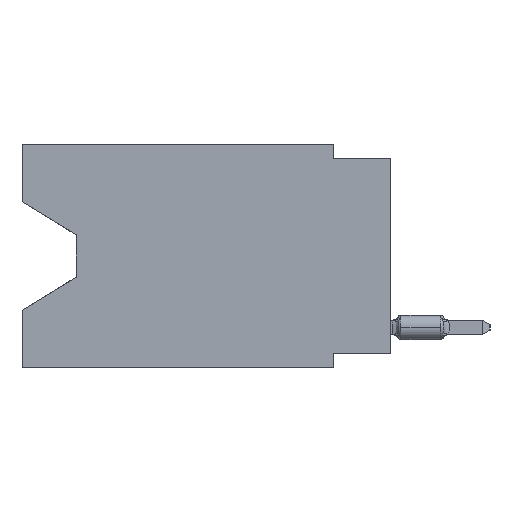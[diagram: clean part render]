
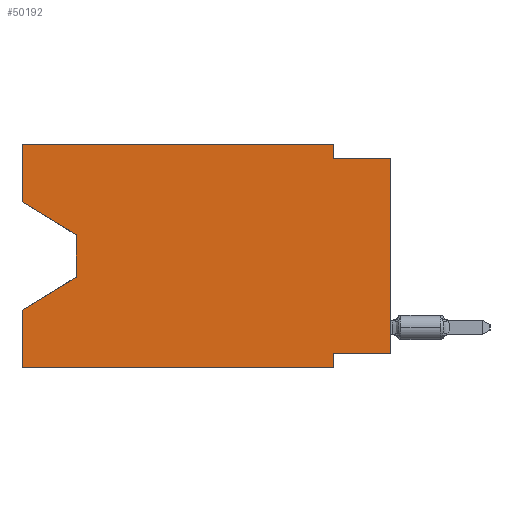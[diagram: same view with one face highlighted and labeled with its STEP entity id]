
A CAD part, left-side view. The second image highlights one B-rep face of the part: STEP entity #50192.
In plain terms, the highlighted planar face has unit normal (-1, 0, 0).
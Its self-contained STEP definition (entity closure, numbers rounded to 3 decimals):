
#1399 = ORIENTED_EDGE ( 'NONE', *, *, #29018, .T. ) ;
#1753 = CARTESIAN_POINT ( 'NONE',  ( 0., 13.97, -5.893 ) ) ;
#2092 = CARTESIAN_POINT ( 'NONE',  ( 0., 16.383, 0. ) ) ;
#2249 = EDGE_CURVE ( 'NONE', #56147, #43736, #60631, .T. ) ;
#2749 = LINE ( 'NONE', #41921, #39977 ) ;
#3584 = AXIS2_PLACEMENT_3D ( 'NONE', #2092, #50902, #56037 ) ;
#4312 = CARTESIAN_POINT ( 'NONE',  ( 0., 2.54, -9.906 ) ) ;
#4635 = VERTEX_POINT ( 'NONE', #38450 ) ;
#6083 = LINE ( 'NONE', #30810, #52205 ) ;
#6683 = DIRECTION ( 'NONE',  ( 0., 0., -1. ) ) ;
#8539 = EDGE_CURVE ( 'NONE', #33124, #56147, #19864, .T. ) ;
#9838 = LINE ( 'NONE', #18857, #56241 ) ;
#11306 = CARTESIAN_POINT ( 'NONE',  ( 0., 2.54, -0.635 ) ) ;
#11333 = CARTESIAN_POINT ( 'NONE',  ( 0., 0., -9.271 ) ) ;
#11708 = FACE_OUTER_BOUND ( 'NONE', #40241, .T. ) ;
#11827 = DIRECTION ( 'NONE',  ( 0., 0., -1. ) ) ;
#11996 = ORIENTED_EDGE ( 'NONE', *, *, #54794, .T. ) ;
#12516 = CARTESIAN_POINT ( 'NONE',  ( 0., 16.383, -9.906 ) ) ;
#13296 = LINE ( 'NONE', #56661, #56611 ) ;
#13859 = EDGE_CURVE ( 'NONE', #33124, #44436, #28386, .T. ) ;
#14690 = ORIENTED_EDGE ( 'NONE', *, *, #31954, .F. ) ;
#15047 = ORIENTED_EDGE ( 'NONE', *, *, #8539, .F. ) ;
#15240 = DIRECTION ( 'NONE',  ( 0., 0.855, -0.519 ) ) ;
#17894 = ORIENTED_EDGE ( 'NONE', *, *, #24638, .F. ) ;
#18492 = CARTESIAN_POINT ( 'NONE',  ( 0., 13.97, -4.013 ) ) ;
#18857 = CARTESIAN_POINT ( 'NONE',  ( 0., 16.383, 0. ) ) ;
#19350 = CARTESIAN_POINT ( 'NONE',  ( 0., 2.54, 0. ) ) ;
#19864 = LINE ( 'NONE', #29501, #58432 ) ;
#20754 = VERTEX_POINT ( 'NONE', #50498 ) ;
#20798 = VERTEX_POINT ( 'NONE', #11306 ) ;
#20839 = CARTESIAN_POINT ( 'NONE',  ( 0., 2.54, -9.906 ) ) ;
#21132 = VECTOR ( 'NONE', #11827, 1000. ) ;
#21393 = CARTESIAN_POINT ( 'NONE',  ( 0., 16.383, -7.36 ) ) ;
#22192 = EDGE_CURVE ( 'NONE', #20798, #44436, #26560, .T. ) ;
#22329 = VERTEX_POINT ( 'NONE', #18492 ) ;
#22827 = VECTOR ( 'NONE', #59502, 1000. ) ;
#23569 = CARTESIAN_POINT ( 'NONE',  ( 0., 0., 0. ) ) ;
#24021 = VECTOR ( 'NONE', #6683, 1000. ) ;
#24364 = VECTOR ( 'NONE', #15240, 1000. ) ;
#24496 = VERTEX_POINT ( 'NONE', #49691 ) ;
#24638 = EDGE_CURVE ( 'NONE', #24496, #25453, #2749, .T. ) ;
#25365 = VERTEX_POINT ( 'NONE', #21393 ) ;
#25453 = VERTEX_POINT ( 'NONE', #19350 ) ;
#25863 = VECTOR ( 'NONE', #52784, 1000. ) ;
#26090 = LINE ( 'NONE', #35089, #22827 ) ;
#26560 = LINE ( 'NONE', #31063, #37861 ) ;
#28386 = LINE ( 'NONE', #23569, #25863 ) ;
#29018 = EDGE_CURVE ( 'NONE', #41207, #25365, #59569, .T. ) ;
#29387 = CARTESIAN_POINT ( 'NONE',  ( 0., 13.97, -5.893 ) ) ;
#29501 = CARTESIAN_POINT ( 'NONE',  ( 0., 0., -9.271 ) ) ;
#30508 = ORIENTED_EDGE ( 'NONE', *, *, #13859, .T. ) ;
#30655 = EDGE_CURVE ( 'NONE', #4635, #25365, #6083, .T. ) ;
#30810 = CARTESIAN_POINT ( 'NONE',  ( 0., 16.383, 0. ) ) ;
#31063 = CARTESIAN_POINT ( 'NONE',  ( 0., 0., -0.635 ) ) ;
#31946 = PLANE ( 'NONE',  #3584 ) ;
#31954 = EDGE_CURVE ( 'NONE', #20754, #24496, #9838, .T. ) ;
#32037 = ORIENTED_EDGE ( 'NONE', *, *, #2249, .F. ) ;
#32900 = DIRECTION ( 'NONE',  ( 0., -0.855, -0.519 ) ) ;
#33124 = VERTEX_POINT ( 'NONE', #11333 ) ;
#35089 = CARTESIAN_POINT ( 'NONE',  ( 0., 2.54, 0. ) ) ;
#35386 = VECTOR ( 'NONE', #42396, 1000. ) ;
#37420 = DIRECTION ( 'NONE',  ( 0., -1., 0. ) ) ;
#37505 = CARTESIAN_POINT ( 'NONE',  ( 0., 13.97, -4.013 ) ) ;
#37546 = ORIENTED_EDGE ( 'NONE', *, *, #56510, .T. ) ;
#37861 = VECTOR ( 'NONE', #51576, 1000. ) ;
#38450 = CARTESIAN_POINT ( 'NONE',  ( 0., 16.383, -9.906 ) ) ;
#39977 = VECTOR ( 'NONE', #37420, 1000. ) ;
#40241 = EDGE_LOOP ( 'NONE', ( #41878, #37546, #1399, #61359, #11996, #32037, #15047, #30508, #50522, #61377, #17894, #14690 ) ) ;
#41207 = VERTEX_POINT ( 'NONE', #1753 ) ;
#41878 = ORIENTED_EDGE ( 'NONE', *, *, #44748, .T. ) ;
#41921 = CARTESIAN_POINT ( 'NONE',  ( 0., 16.383, 0. ) ) ;
#42396 = DIRECTION ( 'NONE',  ( 0., -1., 0. ) ) ;
#43736 = VERTEX_POINT ( 'NONE', #4312 ) ;
#44436 = VERTEX_POINT ( 'NONE', #51685 ) ;
#44748 = EDGE_CURVE ( 'NONE', #20754, #22329, #13296, .T. ) ;
#47602 = EDGE_CURVE ( 'NONE', #25453, #20798, #26090, .T. ) ;
#49118 = DIRECTION ( 'NONE',  ( 0., 0., 1. ) ) ;
#49691 = CARTESIAN_POINT ( 'NONE',  ( 0., 16.383, 0. ) ) ;
#50192 = ADVANCED_FACE ( 'NONE', ( #11708 ), #31946, .F. ) ;
#50498 = CARTESIAN_POINT ( 'NONE',  ( 0., 16.383, -2.546 ) ) ;
#50522 = ORIENTED_EDGE ( 'NONE', *, *, #22192, .F. ) ;
#50902 = DIRECTION ( 'NONE',  ( 1., 0., 0. ) ) ;
#51576 = DIRECTION ( 'NONE',  ( 0., -1., 0. ) ) ;
#51685 = CARTESIAN_POINT ( 'NONE',  ( 0., 0., -0.635 ) ) ;
#52205 = VECTOR ( 'NONE', #49118, 1000. ) ;
#52784 = DIRECTION ( 'NONE',  ( 0., 0., 1. ) ) ;
#54491 = DIRECTION ( 'NONE',  ( 0., 0., 1. ) ) ;
#54794 = EDGE_CURVE ( 'NONE', #4635, #43736, #61660, .T. ) ;
#56037 = DIRECTION ( 'NONE',  ( 0., 0., -1. ) ) ;
#56147 = VERTEX_POINT ( 'NONE', #60502 ) ;
#56241 = VECTOR ( 'NONE', #54491, 1000. ) ;
#56510 = EDGE_CURVE ( 'NONE', #22329, #41207, #56787, .T. ) ;
#56611 = VECTOR ( 'NONE', #32900, 1000. ) ;
#56661 = CARTESIAN_POINT ( 'NONE',  ( 0., 16.383, -2.546 ) ) ;
#56787 = LINE ( 'NONE', #37505, #21132 ) ;
#58432 = VECTOR ( 'NONE', #59996, 1000. ) ;
#59502 = DIRECTION ( 'NONE',  ( 0., 0., -1. ) ) ;
#59569 = LINE ( 'NONE', #29387, #24364 ) ;
#59996 = DIRECTION ( 'NONE',  ( 0., 1., 0. ) ) ;
#60502 = CARTESIAN_POINT ( 'NONE',  ( 0., 2.54, -9.271 ) ) ;
#60631 = LINE ( 'NONE', #20839, #24021 ) ;
#61359 = ORIENTED_EDGE ( 'NONE', *, *, #30655, .F. ) ;
#61377 = ORIENTED_EDGE ( 'NONE', *, *, #47602, .F. ) ;
#61660 = LINE ( 'NONE', #12516, #35386 ) ;
